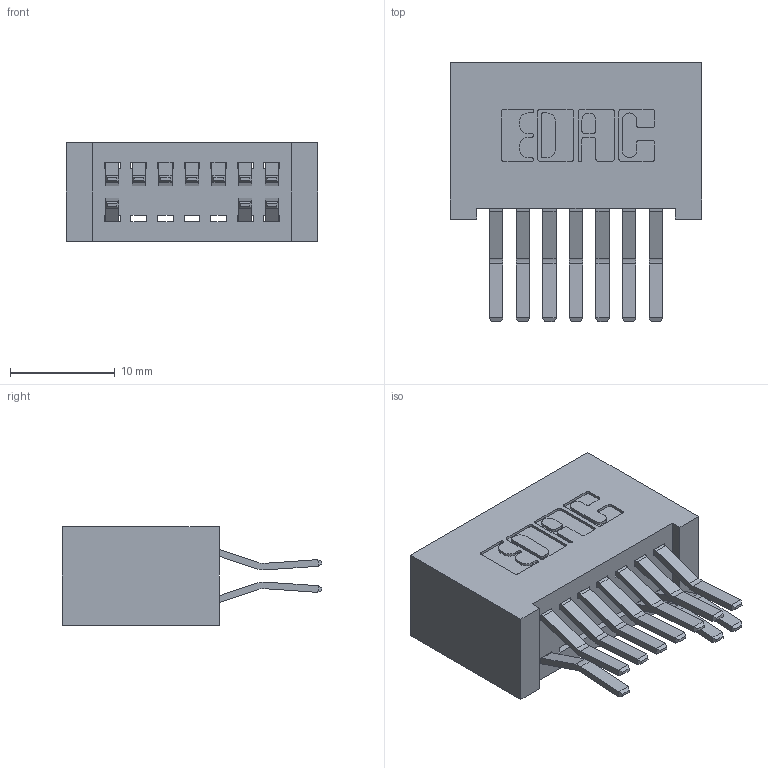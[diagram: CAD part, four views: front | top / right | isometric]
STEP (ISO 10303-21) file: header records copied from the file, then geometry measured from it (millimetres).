
FILE_DESCRIPTION (( 'STEP AP203' ), '1' );
FILE_NAME ('392-014-560-201.STEP', '2018-08-15T00:38:07', ( '' ), ( '' ), 'SwSTEP 2.0', 'SolidWorks 2016', '' );
FILE_SCHEMA (( 'CONFIG_CONTROL_DESIGN' ));
Length unit declared in the file: inch
Products named in the file (3): 342 Part_Lugless; 345-292-001_560 Tail; 392-014-560-201
Assembly tree (11 placements, depth 2):
  392-014-560-201
    342 Part_Lugless
    345-292-001_560 Tail  x10
Bounding box: 24.03 x 24.78 x 9.4 mm (x, y, z)
Volume: 2462.5 mm3; surface area: 3550.5 mm2
Topology: 11 solids, 11 shells, 666 faces, 1969 edges, 1298 vertices
Faces by surface type: plane 446, cylinder 220
Entity records: 8581 total; most frequent: CARTESIAN_POINT 1478, ORIENTED_EDGE 1418, DIRECTION 1317, EDGE_CURVE 709, LINE 585, VECTOR 585, VERTEX_POINT 470, AXIS2_PLACEMENT_3D 366
